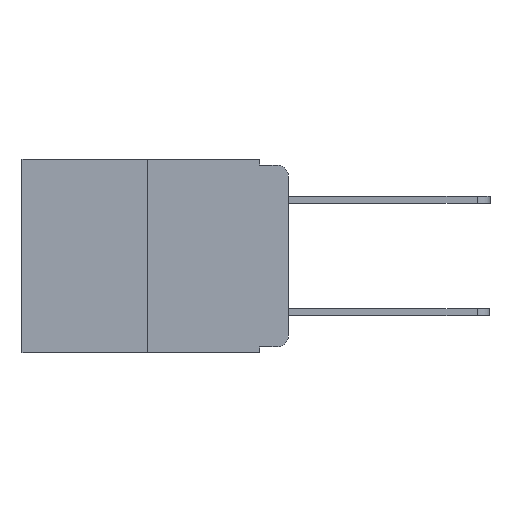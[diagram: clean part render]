
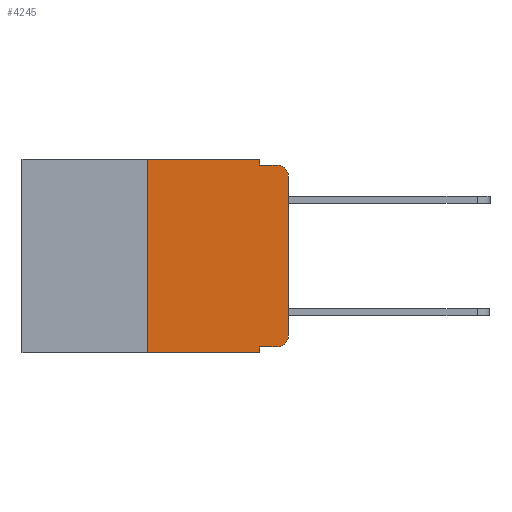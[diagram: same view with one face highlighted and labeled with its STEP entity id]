
A CAD part, left-side view. The second image highlights one B-rep face of the part: STEP entity #4245.
In plain terms, the highlighted planar face has unit normal (-1, 0, 0).
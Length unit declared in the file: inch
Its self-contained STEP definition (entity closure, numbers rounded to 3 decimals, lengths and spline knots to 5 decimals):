
#382 = VECTOR ( 'NONE', #5061, 39.37008 ) ;
#427 = LINE ( 'NONE', #7748, #9017 ) ;
#872 = VERTEX_POINT ( 'NONE', #3620 ) ;
#1007 = VERTEX_POINT ( 'NONE', #18246 ) ;
#1113 = VERTEX_POINT ( 'NONE', #7568 ) ;
#2024 = EDGE_CURVE ( 'NONE', #1007, #12784, #10740, .T. ) ;
#2254 = CARTESIAN_POINT ( 'NONE',  ( 0., 0.051, 0. ) ) ;
#2485 = LINE ( 'NONE', #21103, #11021 ) ;
#3620 = CARTESIAN_POINT ( 'NONE',  ( 0., 0.051, -0.333 ) ) ;
#3667 = ORIENTED_EDGE ( 'NONE', *, *, #2024, .T. ) ;
#3880 = ORIENTED_EDGE ( 'NONE', *, *, #11473, .F. ) ;
#4009 = FACE_OUTER_BOUND ( 'NONE', #15597, .T. ) ;
#4245 = ADVANCED_FACE ( 'NONE', ( #4009 ), #14608, .F. ) ;
#4523 = ORIENTED_EDGE ( 'NONE', *, *, #10435, .T. ) ;
#4700 = AXIS2_PLACEMENT_3D ( 'NONE', #14871, #4826, #16505 ) ;
#4826 = DIRECTION ( 'NONE',  ( -1., 0., 0. ) ) ;
#4933 = ORIENTED_EDGE ( 'NONE', *, *, #6500, .T. ) ;
#5061 = DIRECTION ( 'NONE',  ( 0., 0., 1. ) ) ;
#5122 = CARTESIAN_POINT ( 'NONE',  ( 0., 0.051, -0.01 ) ) ;
#5325 = CARTESIAN_POINT ( 'NONE',  ( 0., 0.02, -0.313 ) ) ;
#5567 = ORIENTED_EDGE ( 'NONE', *, *, #5883, .T. ) ;
#5573 = DIRECTION ( 'NONE',  ( 0., 0., -1. ) ) ;
#5585 = CIRCLE ( 'NONE', #4700, 0.02 ) ;
#5596 = DIRECTION ( 'NONE',  ( 1., 0., 0. ) ) ;
#5883 = EDGE_CURVE ( 'NONE', #872, #7851, #11632, .T. ) ;
#5972 = EDGE_CURVE ( 'NONE', #872, #16515, #10610, .T. ) ;
#6078 = CARTESIAN_POINT ( 'NONE',  ( 0., 0.051, -0.01 ) ) ;
#6337 = ORIENTED_EDGE ( 'NONE', *, *, #8736, .T. ) ;
#6446 = CARTESIAN_POINT ( 'NONE',  ( 0., 0.051, -0.333 ) ) ;
#6500 = EDGE_CURVE ( 'NONE', #7587, #16515, #427, .T. ) ;
#6754 = LINE ( 'NONE', #5122, #19421 ) ;
#6829 = ORIENTED_EDGE ( 'NONE', *, *, #5972, .F. ) ;
#6915 = CARTESIAN_POINT ( 'NONE',  ( 0., 0.25, 0. ) ) ;
#7057 = DIRECTION ( 'NONE',  ( 0., 0., -1. ) ) ;
#7062 = VERTEX_POINT ( 'NONE', #6915 ) ;
#7142 = VECTOR ( 'NONE', #11901, 39.37008 ) ;
#7153 = CARTESIAN_POINT ( 'NONE',  ( 0., 0.02, -0.01 ) ) ;
#7174 = CARTESIAN_POINT ( 'NONE',  ( 0., 0., -0.03 ) ) ;
#7568 = CARTESIAN_POINT ( 'NONE',  ( 0., 0.051, 0. ) ) ;
#7587 = VERTEX_POINT ( 'NONE', #19885 ) ;
#7733 = CARTESIAN_POINT ( 'NONE',  ( 0., 0.473, 0. ) ) ;
#7748 = CARTESIAN_POINT ( 'NONE',  ( 0., 0.473, -0.343 ) ) ;
#7755 = CARTESIAN_POINT ( 'NONE',  ( 0., 0., 0. ) ) ;
#7851 = VERTEX_POINT ( 'NONE', #17302 ) ;
#7860 = CARTESIAN_POINT ( 'NONE',  ( 0., 0.051, -0.343 ) ) ;
#8580 = DIRECTION ( 'NONE',  ( 0., -1., 0. ) ) ;
#8736 = EDGE_CURVE ( 'NONE', #12784, #13416, #5585, .T. ) ;
#9017 = VECTOR ( 'NONE', #20916, 39.37008 ) ;
#9450 = CARTESIAN_POINT ( 'NONE',  ( 0., 0.473, 0. ) ) ;
#10435 = EDGE_CURVE ( 'NONE', #7851, #1007, #15962, .T. ) ;
#10610 = LINE ( 'NONE', #2254, #14953 ) ;
#10740 = LINE ( 'NONE', #7755, #14588 ) ;
#11021 = VECTOR ( 'NONE', #11375, 39.37008 ) ;
#11046 = LINE ( 'NONE', #7733, #18684 ) ;
#11375 = DIRECTION ( 'NONE',  ( 0., 0., -1. ) ) ;
#11473 = EDGE_CURVE ( 'NONE', #7587, #7062, #20979, .T. ) ;
#11554 = ORIENTED_EDGE ( 'NONE', *, *, #12428, .F. ) ;
#11632 = LINE ( 'NONE', #6446, #7142 ) ;
#11901 = DIRECTION ( 'NONE',  ( 0., -1., 0. ) ) ;
#12097 = DIRECTION ( 'NONE',  ( 0., 0., -1. ) ) ;
#12428 = EDGE_CURVE ( 'NONE', #7062, #1113, #11046, .T. ) ;
#12784 = VERTEX_POINT ( 'NONE', #7174 ) ;
#13416 = VERTEX_POINT ( 'NONE', #7153 ) ;
#13467 = CARTESIAN_POINT ( 'NONE',  ( 0., 0.25, 0. ) ) ;
#13843 = ORIENTED_EDGE ( 'NONE', *, *, #17435, .F. ) ;
#14588 = VECTOR ( 'NONE', #21403, 39.37008 ) ;
#14608 = PLANE ( 'NONE',  #19143 ) ;
#14871 = CARTESIAN_POINT ( 'NONE',  ( 0., 0.02, -0.03 ) ) ;
#14953 = VECTOR ( 'NONE', #12097, 39.37008 ) ;
#15597 = EDGE_LOOP ( 'NONE', ( #3667, #6337, #13843, #18936, #11554, #3880, #4933, #6829, #5567, #4523 ) ) ;
#15869 = VERTEX_POINT ( 'NONE', #6078 ) ;
#15962 = CIRCLE ( 'NONE', #19318, 0.02 ) ;
#16505 = DIRECTION ( 'NONE',  ( 0., 0., -1. ) ) ;
#16515 = VERTEX_POINT ( 'NONE', #7860 ) ;
#16982 = DIRECTION ( 'NONE',  ( -1., 0., 0. ) ) ;
#17220 = EDGE_CURVE ( 'NONE', #1113, #15869, #2485, .T. ) ;
#17302 = CARTESIAN_POINT ( 'NONE',  ( 0., 0.02, -0.333 ) ) ;
#17435 = EDGE_CURVE ( 'NONE', #15869, #13416, #6754, .T. ) ;
#18246 = CARTESIAN_POINT ( 'NONE',  ( 0., 0., -0.313 ) ) ;
#18684 = VECTOR ( 'NONE', #19253, 39.37008 ) ;
#18936 = ORIENTED_EDGE ( 'NONE', *, *, #17220, .F. ) ;
#19143 = AXIS2_PLACEMENT_3D ( 'NONE', #9450, #5596, #5573 ) ;
#19253 = DIRECTION ( 'NONE',  ( 0., -1., 0. ) ) ;
#19318 = AXIS2_PLACEMENT_3D ( 'NONE', #5325, #16982, #7057 ) ;
#19421 = VECTOR ( 'NONE', #8580, 39.37008 ) ;
#19885 = CARTESIAN_POINT ( 'NONE',  ( 0., 0.25, -0.343 ) ) ;
#20916 = DIRECTION ( 'NONE',  ( 0., -1., 0. ) ) ;
#20979 = LINE ( 'NONE', #13467, #382 ) ;
#21103 = CARTESIAN_POINT ( 'NONE',  ( 0., 0.051, 0. ) ) ;
#21403 = DIRECTION ( 'NONE',  ( 0., 0., 1. ) ) ;
